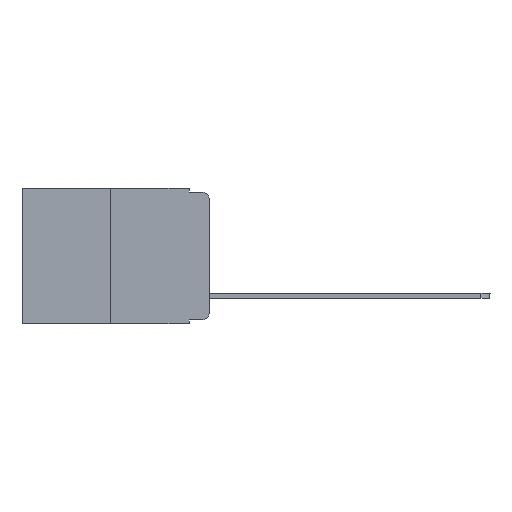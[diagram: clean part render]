
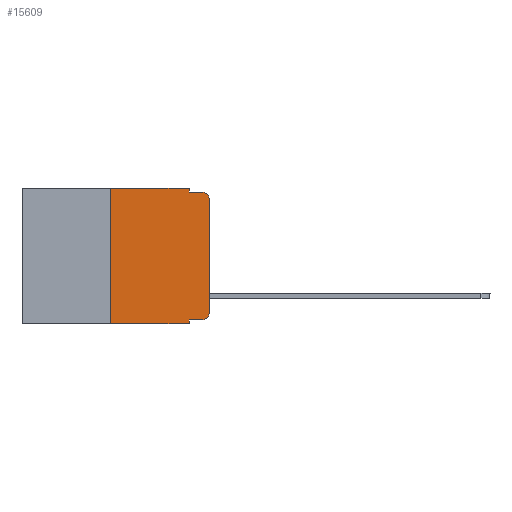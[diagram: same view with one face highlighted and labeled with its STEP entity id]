
A CAD part, left-side view. The second image highlights one B-rep face of the part: STEP entity #15609.
In plain terms, the highlighted planar face has unit normal (-1, 0, 0).
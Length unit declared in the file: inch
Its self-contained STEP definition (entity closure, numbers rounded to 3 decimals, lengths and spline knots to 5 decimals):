
#180 = CARTESIAN_POINT ( 'NONE',  ( 0., 0.051, 0. ) ) ;
#310 = DIRECTION ( 'NONE',  ( 0., -1., 0. ) ) ;
#892 = CARTESIAN_POINT ( 'NONE',  ( 0., 0.051, -0.01 ) ) ;
#899 = VERTEX_POINT ( 'NONE', #1498 ) ;
#1007 = CARTESIAN_POINT ( 'NONE',  ( 0., 0.051, 0. ) ) ;
#1129 = VERTEX_POINT ( 'NONE', #5022 ) ;
#1274 = LINE ( 'NONE', #1007, #3591 ) ;
#1498 = CARTESIAN_POINT ( 'NONE',  ( 0., 0.02, -0.01 ) ) ;
#1590 = LINE ( 'NONE', #4405, #5760 ) ;
#2261 = DIRECTION ( 'NONE',  ( -1., 0., 0. ) ) ;
#2655 = AXIS2_PLACEMENT_3D ( 'NONE', #3678, #2261, #14415 ) ;
#2654 = DIRECTION ( 'NONE',  ( 0., 0., -1. ) ) ;
#3300 = VECTOR ( 'NONE', #17264, 39.37008 ) ;
#3340 = LINE ( 'NONE', #17339, #9637 ) ;
#3401 = VECTOR ( 'NONE', #5697, 39.37008 ) ;
#3591 = VECTOR ( 'NONE', #7539, 39.37008 ) ;
#3678 = CARTESIAN_POINT ( 'NONE',  ( 0., 0.02, -0.313 ) ) ;
#3753 = CARTESIAN_POINT ( 'NONE',  ( 0., 0.02, -0.03 ) ) ;
#3833 = VERTEX_POINT ( 'NONE', #9314 ) ;
#3957 = EDGE_CURVE ( 'NONE', #7397, #7711, #1590, .T. ) ;
#4021 = CARTESIAN_POINT ( 'NONE',  ( 0., 0.473, 0. ) ) ;
#4405 = CARTESIAN_POINT ( 'NONE',  ( 0., 0.051, -0.333 ) ) ;
#4871 = LINE ( 'NONE', #9056, #7146 ) ;
#4988 = ORIENTED_EDGE ( 'NONE', *, *, #10605, .F. ) ;
#5022 = CARTESIAN_POINT ( 'NONE',  ( 0., 0.051, -0.343 ) ) ;
#5105 = DIRECTION ( 'NONE',  ( -1., 0., 0. ) ) ;
#5131 = ORIENTED_EDGE ( 'NONE', *, *, #10448, .F. ) ;
#5363 = CARTESIAN_POINT ( 'NONE',  ( 0., 0.051, 0. ) ) ;
#5697 = DIRECTION ( 'NONE',  ( 0., 0., -1. ) ) ;
#5760 = VECTOR ( 'NONE', #310, 39.37008 ) ;
#5831 = AXIS2_PLACEMENT_3D ( 'NONE', #13234, #8006, #2654 ) ;
#6383 = ORIENTED_EDGE ( 'NONE', *, *, #12794, .T. ) ;
#7065 = VECTOR ( 'NONE', #16082, 39.37008 ) ;
#7146 = VECTOR ( 'NONE', #15512, 39.37008 ) ;
#7299 = VERTEX_POINT ( 'NONE', #11106 ) ;
#7397 = VERTEX_POINT ( 'NONE', #12719 ) ;
#7460 = VERTEX_POINT ( 'NONE', #11505 ) ;
#7539 = DIRECTION ( 'NONE',  ( 0., 0., -1. ) ) ;
#7608 = AXIS2_PLACEMENT_3D ( 'NONE', #3753, #5105, #14430 ) ;
#7711 = VERTEX_POINT ( 'NONE', #14540 ) ;
#8006 = DIRECTION ( 'NONE',  ( 1., 0., 0. ) ) ;
#8304 = VERTEX_POINT ( 'NONE', #13341 ) ;
#8948 = DIRECTION ( 'NONE',  ( 0., -1., 0. ) ) ;
#8985 = LINE ( 'NONE', #4021, #7065 ) ;
#9056 = CARTESIAN_POINT ( 'NONE',  ( 0., 0.25, 0. ) ) ;
#9314 = CARTESIAN_POINT ( 'NONE',  ( 0., 0., -0.03 ) ) ;
#9637 = VECTOR ( 'NONE', #13407, 39.37008 ) ;
#10245 = ORIENTED_EDGE ( 'NONE', *, *, #11313, .T. ) ;
#10334 = ORIENTED_EDGE ( 'NONE', *, *, #12246, .T. ) ;
#10448 = EDGE_CURVE ( 'NONE', #15502, #8304, #15101, .T. ) ;
#10605 = EDGE_CURVE ( 'NONE', #16022, #7299, #4871, .T. ) ;
#10613 = FACE_OUTER_BOUND ( 'NONE', #11195, .T. ) ;
#10627 = EDGE_CURVE ( 'NONE', #7397, #1129, #1274, .T. ) ;
#11106 = CARTESIAN_POINT ( 'NONE',  ( 0., 0.25, 0. ) ) ;
#11125 = VECTOR ( 'NONE', #8948, 39.37008 ) ;
#11157 = ORIENTED_EDGE ( 'NONE', *, *, #14433, .F. ) ;
#11195 = EDGE_LOOP ( 'NONE', ( #6383, #10245, #15499, #5131, #11157, #4988, #10334, #13109, #14904, #13492 ) ) ;
#11313 = EDGE_CURVE ( 'NONE', #3833, #899, #11695, .T. ) ;
#11478 = CIRCLE ( 'NONE', #2655, 0.02 ) ;
#11505 = CARTESIAN_POINT ( 'NONE',  ( 0., 0., -0.313 ) ) ;
#11695 = CIRCLE ( 'NONE', #7608, 0.02 ) ;
#12059 = EDGE_CURVE ( 'NONE', #7711, #7460, #11478, .T. ) ;
#12111 = CARTESIAN_POINT ( 'NONE',  ( 0., 0., 0. ) ) ;
#12246 = EDGE_CURVE ( 'NONE', #16022, #1129, #3340, .T. ) ;
#12719 = CARTESIAN_POINT ( 'NONE',  ( 0., 0.051, -0.333 ) ) ;
#12794 = EDGE_CURVE ( 'NONE', #7460, #3833, #17319, .T. ) ;
#13109 = ORIENTED_EDGE ( 'NONE', *, *, #10627, .F. ) ;
#13226 = EDGE_CURVE ( 'NONE', #8304, #899, #14889, .T. ) ;
#13234 = CARTESIAN_POINT ( 'NONE',  ( 0., 0.473, 0. ) ) ;
#13341 = CARTESIAN_POINT ( 'NONE',  ( 0., 0.051, -0.01 ) ) ;
#13407 = DIRECTION ( 'NONE',  ( 0., -1., 0. ) ) ;
#13492 = ORIENTED_EDGE ( 'NONE', *, *, #12059, .T. ) ;
#14033 = CARTESIAN_POINT ( 'NONE',  ( 0., 0.25, -0.343 ) ) ;
#14415 = DIRECTION ( 'NONE',  ( 0., 0., -1. ) ) ;
#14430 = DIRECTION ( 'NONE',  ( 0., 0., -1. ) ) ;
#14433 = EDGE_CURVE ( 'NONE', #7299, #15502, #8985, .T. ) ;
#14540 = CARTESIAN_POINT ( 'NONE',  ( 0., 0.02, -0.333 ) ) ;
#14889 = LINE ( 'NONE', #892, #11125 ) ;
#14904 = ORIENTED_EDGE ( 'NONE', *, *, #3957, .T. ) ;
#15101 = LINE ( 'NONE', #180, #3401 ) ;
#15499 = ORIENTED_EDGE ( 'NONE', *, *, #13226, .F. ) ;
#15502 = VERTEX_POINT ( 'NONE', #5363 ) ;
#15512 = DIRECTION ( 'NONE',  ( 0., 0., 1. ) ) ;
#15609 = ADVANCED_FACE ( 'NONE', ( #10613 ), #17213, .F. ) ;
#16022 = VERTEX_POINT ( 'NONE', #14033 ) ;
#16082 = DIRECTION ( 'NONE',  ( 0., -1., 0. ) ) ;
#17213 = PLANE ( 'NONE',  #5831 ) ;
#17264 = DIRECTION ( 'NONE',  ( 0., 0., 1. ) ) ;
#17319 = LINE ( 'NONE', #12111, #3300 ) ;
#17339 = CARTESIAN_POINT ( 'NONE',  ( 0., 0.473, -0.343 ) ) ;
